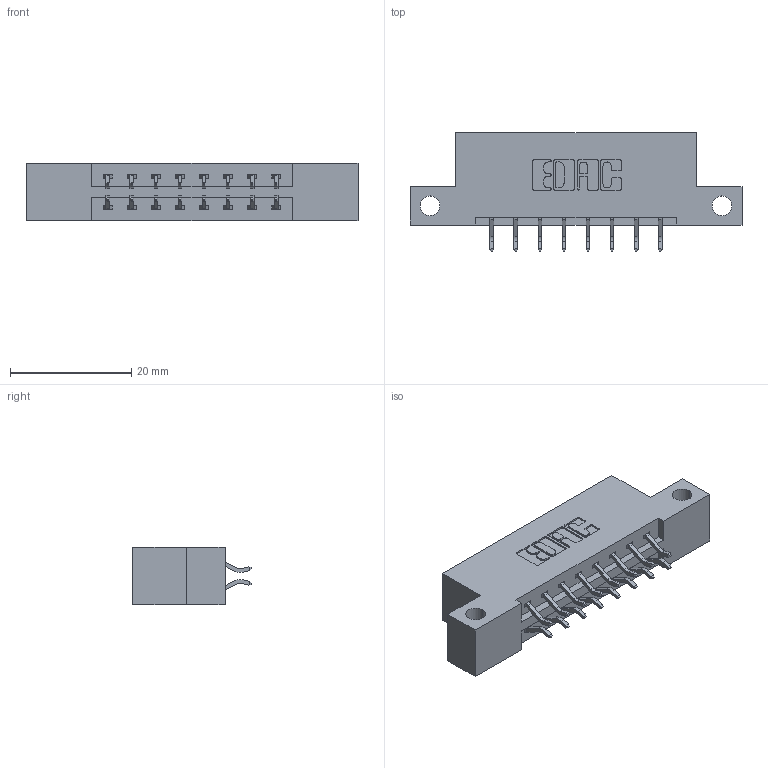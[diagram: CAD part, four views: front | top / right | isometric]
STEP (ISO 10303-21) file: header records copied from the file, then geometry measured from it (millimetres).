
FILE_DESCRIPTION (( 'STEP AP203' ), '1' );
FILE_NAME ('387-016-556-212.STEP', '2019-10-15T23:48:14', ( '' ), ( '' ), 'SwSTEP 2.0', 'SolidWorks 2016', '' );
FILE_SCHEMA (( 'CONFIG_CONTROL_DESIGN' ));
Length unit declared in the file: inch
Products named in the file (3): 387-016-556-212; 345-292-001_556 Tail; 337 Part_Flush Mounting Lugs - Side Mount
Assembly tree (17 placements, depth 2):
  387-016-556-212
    337 Part_Flush Mounting Lugs - Side Mount
    345-292-001_556 Tail  x16
Bounding box: 54.71 x 19.57 x 9.4 mm (x, y, z)
Volume: 5225.4 mm3; surface area: 5407 mm2
Topology: 17 solids, 17 shells, 1074 faces, 3175 edges, 2094 vertices
Faces by surface type: plane 742, cylinder 332
Entity records: 10823 total; most frequent: CARTESIAN_POINT 1866, ORIENTED_EDGE 1790, DIRECTION 1639, EDGE_CURVE 895, VECTOR 759, LINE 759, VERTEX_POINT 594, AXIS2_PLACEMENT_3D 440
